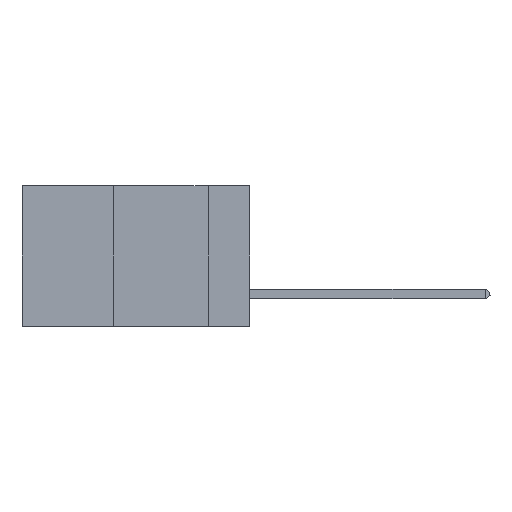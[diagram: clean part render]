
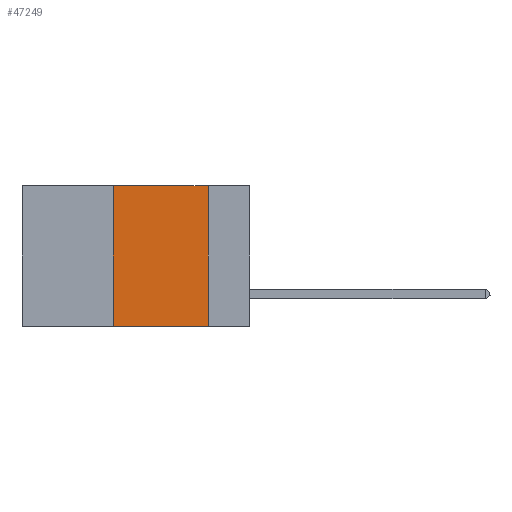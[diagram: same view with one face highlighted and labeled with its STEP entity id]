
A CAD part, left-side view. The second image highlights one B-rep face of the part: STEP entity #47249.
In plain terms, the highlighted planar face has unit normal (-1, 0, 0).
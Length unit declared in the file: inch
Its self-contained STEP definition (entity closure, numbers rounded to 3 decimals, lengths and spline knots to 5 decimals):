
#1155 = VERTEX_POINT ( 'NONE', #36342 ) ;
#1594 = ORIENTED_EDGE ( 'NONE', *, *, #12385, .F. ) ;
#3648 = ORIENTED_EDGE ( 'NONE', *, *, #5535, .F. ) ;
#4765 = CARTESIAN_POINT ( 'NONE',  ( 0., 0.36, 0. ) ) ;
#5535 = EDGE_CURVE ( 'NONE', #21818, #1155, #29058, .T. ) ;
#6211 = VECTOR ( 'NONE', #31328, 39.37008 ) ;
#7543 = CARTESIAN_POINT ( 'NONE',  ( 0., 0.36, -0.37 ) ) ;
#8153 = DIRECTION ( 'NONE',  ( 1., 0., 0. ) ) ;
#8607 = EDGE_LOOP ( 'NONE', ( #31572, #3648, #1594, #24632 ) ) ;
#10291 = CARTESIAN_POINT ( 'NONE',  ( 0., 0.11, -0.37 ) ) ;
#11176 = EDGE_CURVE ( 'NONE', #45466, #39420, #27156, .T. ) ;
#11749 = CARTESIAN_POINT ( 'NONE',  ( 0., 0.6, -0.37 ) ) ;
#12385 = EDGE_CURVE ( 'NONE', #45466, #21818, #13213, .T. ) ;
#13213 = LINE ( 'NONE', #40740, #34187 ) ;
#15865 = AXIS2_PLACEMENT_3D ( 'NONE', #27231, #8153, #34914 ) ;
#21818 = VERTEX_POINT ( 'NONE', #4765 ) ;
#23280 = DIRECTION ( 'NONE',  ( 0., 0., -1. ) ) ;
#24632 = ORIENTED_EDGE ( 'NONE', *, *, #11176, .T. ) ;
#26419 = VECTOR ( 'NONE', #23280, 39.37008 ) ;
#27156 = LINE ( 'NONE', #11749, #6211 ) ;
#27231 = CARTESIAN_POINT ( 'NONE',  ( 0., 0.6, 0. ) ) ;
#29058 = LINE ( 'NONE', #34501, #48940 ) ;
#31328 = DIRECTION ( 'NONE',  ( 0., -1., 0. ) ) ;
#31572 = ORIENTED_EDGE ( 'NONE', *, *, #49454, .F. ) ;
#33250 = FACE_OUTER_BOUND ( 'NONE', #8607, .T. ) ;
#34120 = CARTESIAN_POINT ( 'NONE',  ( 0., 0.11, 0. ) ) ;
#34187 = VECTOR ( 'NONE', #44619, 39.37008 ) ;
#34501 = CARTESIAN_POINT ( 'NONE',  ( 0., 0.6, 0. ) ) ;
#34914 = DIRECTION ( 'NONE',  ( 0., 0., -1. ) ) ;
#36342 = CARTESIAN_POINT ( 'NONE',  ( 0., 0.11, 0. ) ) ;
#36607 = LINE ( 'NONE', #34120, #26419 ) ;
#39420 = VERTEX_POINT ( 'NONE', #10291 ) ;
#40740 = CARTESIAN_POINT ( 'NONE',  ( 0., 0.36, 0. ) ) ;
#42265 = DIRECTION ( 'NONE',  ( 0., -1., 0. ) ) ;
#42503 = PLANE ( 'NONE',  #15865 ) ;
#44619 = DIRECTION ( 'NONE',  ( 0., 0., 1. ) ) ;
#45466 = VERTEX_POINT ( 'NONE', #7543 ) ;
#47249 = ADVANCED_FACE ( 'NONE', ( #33250 ), #42503, .F. ) ;
#48940 = VECTOR ( 'NONE', #42265, 39.37008 ) ;
#49454 = EDGE_CURVE ( 'NONE', #1155, #39420, #36607, .T. ) ;
